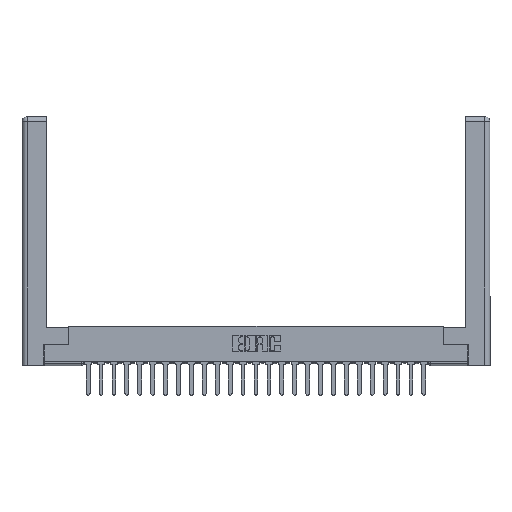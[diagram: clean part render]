
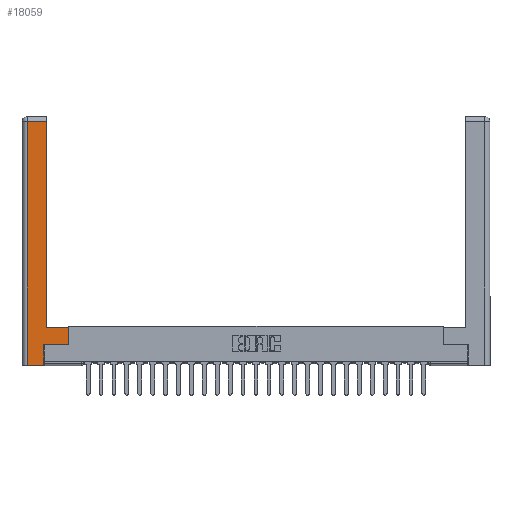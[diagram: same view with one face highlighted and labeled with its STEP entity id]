
A CAD part, top view. The second image highlights one B-rep face of the part: STEP entity #18059.
In plain terms, the highlighted planar face has unit normal (0, 0, 1).
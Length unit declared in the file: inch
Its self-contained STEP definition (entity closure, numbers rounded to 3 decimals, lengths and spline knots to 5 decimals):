
#342 = FACE_OUTER_BOUND ( 'NONE', #25791, .T. ) ;
#1044 = DIRECTION ( 'NONE',  ( -1., 0., 0. ) ) ;
#1635 = CARTESIAN_POINT ( 'NONE',  ( 0.265, 0., 0. ) ) ;
#1637 = ORIENTED_EDGE ( 'NONE', *, *, #12258, .T. ) ;
#3148 = VECTOR ( 'NONE', #18450, 39.37008 ) ;
#3371 = LINE ( 'NONE', #14591, #17110 ) ;
#5039 = DIRECTION ( 'NONE',  ( 0., -1., 0. ) ) ;
#5596 = LINE ( 'NONE', #1635, #23810 ) ;
#5715 = CARTESIAN_POINT ( 'NONE',  ( 0.0615, 2.94, 0. ) ) ;
#6467 = EDGE_CURVE ( 'NONE', #10953, #8128, #5596, .T. ) ;
#7093 = EDGE_CURVE ( 'NONE', #26672, #21808, #21348, .T. ) ;
#8128 = VERTEX_POINT ( 'NONE', #18807 ) ;
#8270 = DIRECTION ( 'NONE',  ( 0., 1., 0. ) ) ;
#8979 = DIRECTION ( 'NONE',  ( 0., 1., 0. ) ) ;
#9625 = EDGE_CURVE ( 'NONE', #8128, #17777, #24635, .T. ) ;
#10001 = LINE ( 'NONE', #16774, #15777 ) ;
#10032 = CARTESIAN_POINT ( 'NONE',  ( 0.295, 2.94, 0. ) ) ;
#10043 = VERTEX_POINT ( 'NONE', #12662 ) ;
#10047 = DIRECTION ( 'NONE',  ( -1., 0., 0. ) ) ;
#10906 = VECTOR ( 'NONE', #8979, 39.37008 ) ;
#10953 = VERTEX_POINT ( 'NONE', #18045 ) ;
#11748 = LINE ( 'NONE', #15853, #3148 ) ;
#12258 = EDGE_CURVE ( 'NONE', #17777, #26672, #11748, .T. ) ;
#12662 = CARTESIAN_POINT ( 'NONE',  ( 0.0615, 2.94, 0. ) ) ;
#13963 = VECTOR ( 'NONE', #10047, 39.37008 ) ;
#14393 = ORIENTED_EDGE ( 'NONE', *, *, #15932, .T. ) ;
#14519 = EDGE_CURVE ( 'NONE', #10043, #10953, #21618, .T. ) ;
#14591 = CARTESIAN_POINT ( 'NONE',  ( 0.295, 0.45, 0. ) ) ;
#15381 = CARTESIAN_POINT ( 'NONE',  ( 0.295, 0.45, 0. ) ) ;
#15777 = VECTOR ( 'NONE', #8270, 39.37008 ) ;
#15823 = AXIS2_PLACEMENT_3D ( 'NONE', #22555, #25163, #1044 ) ;
#15839 = CARTESIAN_POINT ( 'NONE',  ( 0.265, 0.245, 0. ) ) ;
#15853 = CARTESIAN_POINT ( 'NONE',  ( 0.565, 0.245, 0. ) ) ;
#15891 = ORIENTED_EDGE ( 'NONE', *, *, #20308, .T. ) ;
#15932 = EDGE_CURVE ( 'NONE', #24403, #27053, #10001, .T. ) ;
#16320 = ORIENTED_EDGE ( 'NONE', *, *, #14519, .T. ) ;
#16774 = CARTESIAN_POINT ( 'NONE',  ( 0.295, 3., 0. ) ) ;
#16879 = VECTOR ( 'NONE', #24102, 39.37008 ) ;
#17110 = VECTOR ( 'NONE', #28152, 39.37008 ) ;
#17193 = DIRECTION ( 'NONE',  ( 1., 0., 0. ) ) ;
#17324 = ORIENTED_EDGE ( 'NONE', *, *, #24176, .T. ) ;
#17615 = CARTESIAN_POINT ( 'NONE',  ( 0.565, 0.245, 0. ) ) ;
#17657 = ORIENTED_EDGE ( 'NONE', *, *, #6467, .T. ) ;
#17777 = VERTEX_POINT ( 'NONE', #21230 ) ;
#18045 = CARTESIAN_POINT ( 'NONE',  ( 0.0615, 0., 0. ) ) ;
#18059 = ADVANCED_FACE ( 'NONE', ( #342 ), #20622, .F. ) ;
#18164 = VECTOR ( 'NONE', #5039, 39.37008 ) ;
#18450 = DIRECTION ( 'NONE',  ( 1., 0., 0. ) ) ;
#18807 = CARTESIAN_POINT ( 'NONE',  ( 0.265, 0., 0. ) ) ;
#19658 = CARTESIAN_POINT ( 'NONE',  ( 0.565, 0.45, 0. ) ) ;
#20308 = EDGE_CURVE ( 'NONE', #21808, #24403, #3371, .T. ) ;
#20583 = CARTESIAN_POINT ( 'NONE',  ( 0.0615, 0., 0. ) ) ;
#20622 = PLANE ( 'NONE',  #15823 ) ;
#21230 = CARTESIAN_POINT ( 'NONE',  ( 0.265, 0.245, 0. ) ) ;
#21348 = LINE ( 'NONE', #19658, #16879 ) ;
#21618 = LINE ( 'NONE', #20583, #18164 ) ;
#21808 = VERTEX_POINT ( 'NONE', #22029 ) ;
#22029 = CARTESIAN_POINT ( 'NONE',  ( 0.565, 0.45, 0. ) ) ;
#22555 = CARTESIAN_POINT ( 'NONE',  ( 0., 0., 0. ) ) ;
#22559 = LINE ( 'NONE', #5715, #13963 ) ;
#23803 = ORIENTED_EDGE ( 'NONE', *, *, #9625, .T. ) ;
#23810 = VECTOR ( 'NONE', #17193, 39.37008 ) ;
#24102 = DIRECTION ( 'NONE',  ( 0., 1., 0. ) ) ;
#24176 = EDGE_CURVE ( 'NONE', #27053, #10043, #22559, .T. ) ;
#24403 = VERTEX_POINT ( 'NONE', #15381 ) ;
#24635 = LINE ( 'NONE', #15839, #10906 ) ;
#25044 = ORIENTED_EDGE ( 'NONE', *, *, #7093, .T. ) ;
#25163 = DIRECTION ( 'NONE',  ( 0., 0., -1. ) ) ;
#25791 = EDGE_LOOP ( 'NONE', ( #14393, #17324, #16320, #17657, #23803, #1637, #25044, #15891 ) ) ;
#26672 = VERTEX_POINT ( 'NONE', #17615 ) ;
#27053 = VERTEX_POINT ( 'NONE', #10032 ) ;
#28152 = DIRECTION ( 'NONE',  ( -1., 0., 0. ) ) ;
